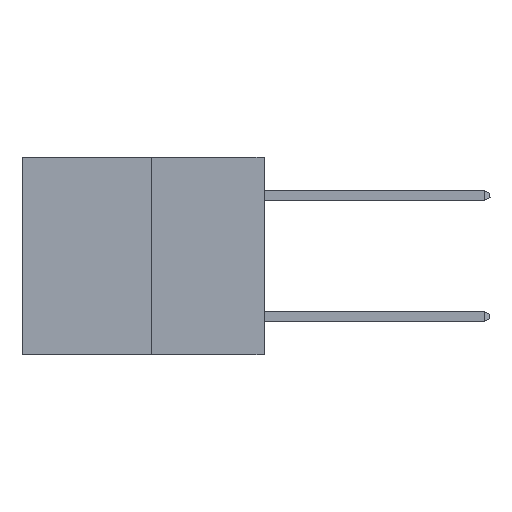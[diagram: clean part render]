
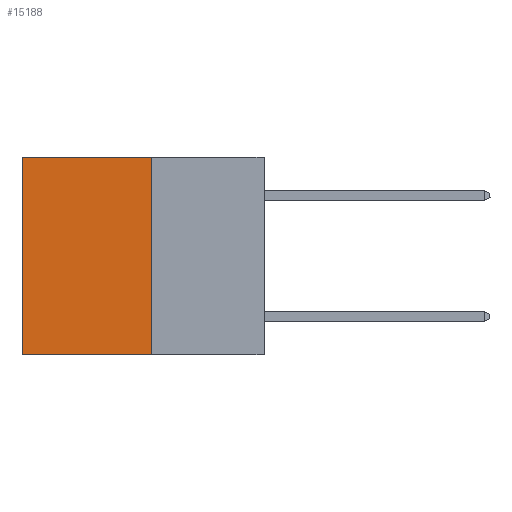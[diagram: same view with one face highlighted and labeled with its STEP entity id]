
A CAD part, left-side view. The second image highlights one B-rep face of the part: STEP entity #15188.
In plain terms, the highlighted planar face has unit normal (-1, 0, 0).
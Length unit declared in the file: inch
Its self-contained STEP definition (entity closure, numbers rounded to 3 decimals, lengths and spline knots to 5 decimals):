
#240 = VECTOR ( 'NONE', #19843, 39.37008 ) ;
#395 = DIRECTION ( 'NONE',  ( 0., 1., 0. ) ) ;
#1061 = VECTOR ( 'NONE', #22920, 39.37008 ) ;
#1067 = PLANE ( 'NONE',  #16421 ) ;
#1140 = VERTEX_POINT ( 'NONE', #22737 ) ;
#1197 = EDGE_CURVE ( 'NONE', #19330, #15195, #19032, .T. ) ;
#1281 = EDGE_CURVE ( 'NONE', #1140, #19848, #11405, .T. ) ;
#1384 = ORIENTED_EDGE ( 'NONE', *, *, #26502, .F. ) ;
#2869 = CARTESIAN_POINT ( 'NONE',  ( 0.3165, 0.28, -0.49 ) ) ;
#3675 = EDGE_CURVE ( 'NONE', #19848, #15195, #6114, .T. ) ;
#4596 = ORIENTED_EDGE ( 'NONE', *, *, #1281, .T. ) ;
#4925 = CARTESIAN_POINT ( 'NONE',  ( 0.3165, 0.28, 0. ) ) ;
#5079 = ORIENTED_EDGE ( 'NONE', *, *, #1197, .F. ) ;
#5807 = CARTESIAN_POINT ( 'NONE',  ( 0.3165, 0.28, -0.49 ) ) ;
#6114 = LINE ( 'NONE', #26507, #240 ) ;
#7243 = LINE ( 'NONE', #22715, #1061 ) ;
#7293 = FACE_OUTER_BOUND ( 'NONE', #9060, .T. ) ;
#9060 = EDGE_LOOP ( 'NONE', ( #11483, #5079, #1384, #4596 ) ) ;
#10021 = VECTOR ( 'NONE', #20975, 39.37008 ) ;
#11405 = LINE ( 'NONE', #4925, #10021 ) ;
#11483 = ORIENTED_EDGE ( 'NONE', *, *, #3675, .T. ) ;
#12097 = VECTOR ( 'NONE', #395, 39.37008 ) ;
#14205 = CARTESIAN_POINT ( 'NONE',  ( 0.3165, 0.6, -0.49 ) ) ;
#15188 = ADVANCED_FACE ( 'NONE', ( #7293 ), #1067, .F. ) ;
#15195 = VERTEX_POINT ( 'NONE', #14205 ) ;
#16421 = AXIS2_PLACEMENT_3D ( 'NONE', #5807, #21260, #25216 ) ;
#17470 = CARTESIAN_POINT ( 'NONE',  ( 0.3165, 0.6, 0. ) ) ;
#19032 = LINE ( 'NONE', #2869, #12097 ) ;
#19330 = VERTEX_POINT ( 'NONE', #26970 ) ;
#19843 = DIRECTION ( 'NONE',  ( 0., 0., -1. ) ) ;
#19848 = VERTEX_POINT ( 'NONE', #17470 ) ;
#20975 = DIRECTION ( 'NONE',  ( 0., 1., 0. ) ) ;
#21260 = DIRECTION ( 'NONE',  ( 1., 0., 0. ) ) ;
#22715 = CARTESIAN_POINT ( 'NONE',  ( 0.3165, 0.28, -0.49 ) ) ;
#22737 = CARTESIAN_POINT ( 'NONE',  ( 0.3165, 0.28, 0. ) ) ;
#22920 = DIRECTION ( 'NONE',  ( 0., 0., -1. ) ) ;
#25216 = DIRECTION ( 'NONE',  ( 0., 0., -1. ) ) ;
#26502 = EDGE_CURVE ( 'NONE', #1140, #19330, #7243, .T. ) ;
#26507 = CARTESIAN_POINT ( 'NONE',  ( 0.3165, 0.6, -0.49 ) ) ;
#26970 = CARTESIAN_POINT ( 'NONE',  ( 0.3165, 0.28, -0.49 ) ) ;
